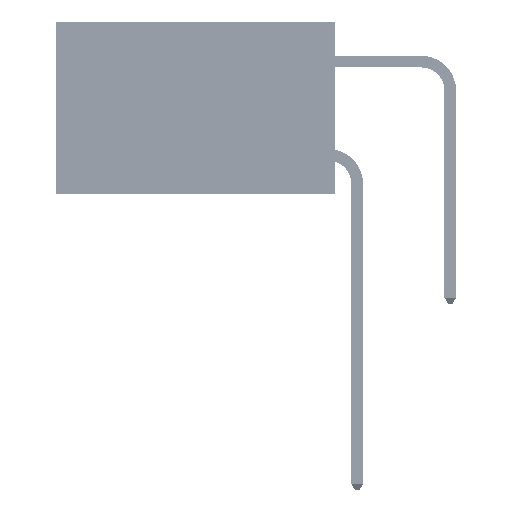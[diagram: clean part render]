
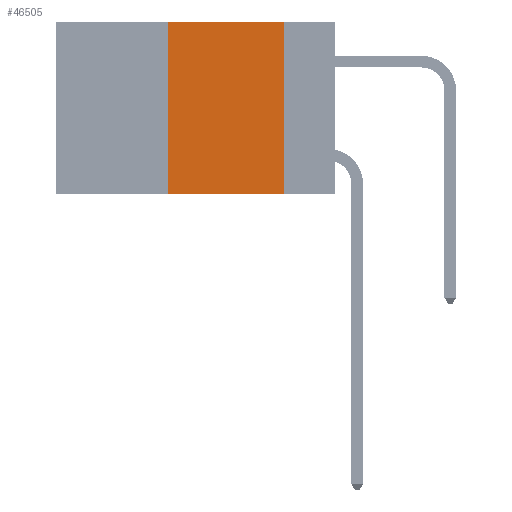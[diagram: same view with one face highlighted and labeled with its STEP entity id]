
A CAD part, left-side view. The second image highlights one B-rep face of the part: STEP entity #46505.
In plain terms, the highlighted planar face has unit normal (-1, 0, 0).
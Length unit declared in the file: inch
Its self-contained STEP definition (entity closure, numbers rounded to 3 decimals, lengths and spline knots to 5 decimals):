
#631 = VECTOR ( 'NONE', #42980, 39.37008 ) ;
#8178 = DIRECTION ( 'NONE',  ( 0., 0., -1. ) ) ;
#10918 = EDGE_CURVE ( 'NONE', #52552, #21413, #40347, .T. ) ;
#11039 = CARTESIAN_POINT ( 'NONE',  ( 0., 0.11, -0.37 ) ) ;
#11431 = CARTESIAN_POINT ( 'NONE',  ( 0., 0.36, 0. ) ) ;
#12648 = PLANE ( 'NONE',  #35776 ) ;
#14059 = DIRECTION ( 'NONE',  ( 0., -1., 0. ) ) ;
#15893 = CARTESIAN_POINT ( 'NONE',  ( 0., 0.6, 0. ) ) ;
#15950 = VERTEX_POINT ( 'NONE', #25081 ) ;
#16246 = DIRECTION ( 'NONE',  ( 1., 0., 0. ) ) ;
#20377 = VECTOR ( 'NONE', #32008, 39.37008 ) ;
#20723 = LINE ( 'NONE', #21067, #39329 ) ;
#21067 = CARTESIAN_POINT ( 'NONE',  ( 0., 0.11, 0. ) ) ;
#21413 = VERTEX_POINT ( 'NONE', #40231 ) ;
#22418 = ORIENTED_EDGE ( 'NONE', *, *, #51563, .F. ) ;
#22834 = ORIENTED_EDGE ( 'NONE', *, *, #24200, .F. ) ;
#24200 = EDGE_CURVE ( 'NONE', #15950, #52552, #35739, .T. ) ;
#24599 = VECTOR ( 'NONE', #14059, 39.37008 ) ;
#25081 = CARTESIAN_POINT ( 'NONE',  ( 0., 0.36, -0.37 ) ) ;
#26753 = CARTESIAN_POINT ( 'NONE',  ( 0., 0.6, 0. ) ) ;
#28166 = FACE_OUTER_BOUND ( 'NONE', #29198, .T. ) ;
#28456 = DIRECTION ( 'NONE',  ( 0., 0., -1. ) ) ;
#29198 = EDGE_LOOP ( 'NONE', ( #22418, #33606, #22834, #33677 ) ) ;
#32008 = DIRECTION ( 'NONE',  ( 0., 0., 1. ) ) ;
#32774 = EDGE_CURVE ( 'NONE', #15950, #36275, #35515, .T. ) ;
#33606 = ORIENTED_EDGE ( 'NONE', *, *, #10918, .F. ) ;
#33677 = ORIENTED_EDGE ( 'NONE', *, *, #32774, .T. ) ;
#35515 = LINE ( 'NONE', #38949, #24599 ) ;
#35739 = LINE ( 'NONE', #51670, #20377 ) ;
#35776 = AXIS2_PLACEMENT_3D ( 'NONE', #15893, #16246, #28456 ) ;
#36275 = VERTEX_POINT ( 'NONE', #11039 ) ;
#38949 = CARTESIAN_POINT ( 'NONE',  ( 0., 0.6, -0.37 ) ) ;
#39329 = VECTOR ( 'NONE', #8178, 39.37008 ) ;
#40231 = CARTESIAN_POINT ( 'NONE',  ( 0., 0.11, 0. ) ) ;
#40347 = LINE ( 'NONE', #26753, #631 ) ;
#42980 = DIRECTION ( 'NONE',  ( 0., -1., 0. ) ) ;
#46505 = ADVANCED_FACE ( 'NONE', ( #28166 ), #12648, .F. ) ;
#51563 = EDGE_CURVE ( 'NONE', #21413, #36275, #20723, .T. ) ;
#51670 = CARTESIAN_POINT ( 'NONE',  ( 0., 0.36, 0. ) ) ;
#52552 = VERTEX_POINT ( 'NONE', #11431 ) ;
